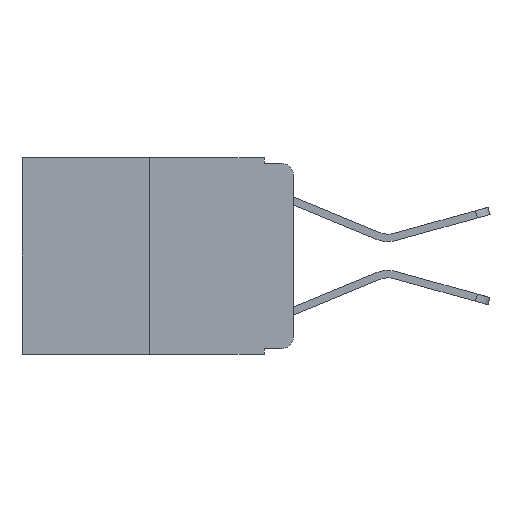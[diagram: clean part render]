
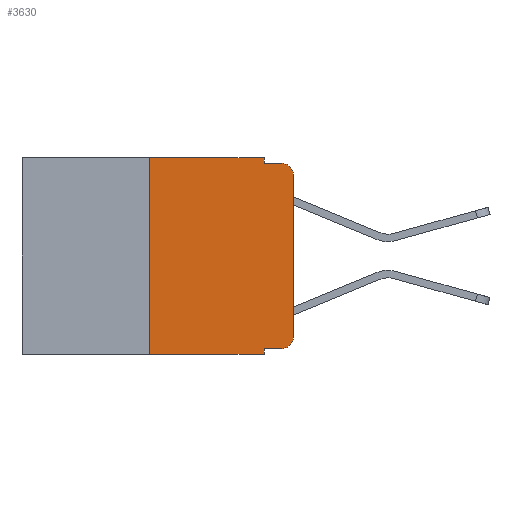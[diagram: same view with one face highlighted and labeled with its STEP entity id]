
A CAD part, left-side view. The second image highlights one B-rep face of the part: STEP entity #3630.
In plain terms, the highlighted planar face has unit normal (-1, 0, 0).
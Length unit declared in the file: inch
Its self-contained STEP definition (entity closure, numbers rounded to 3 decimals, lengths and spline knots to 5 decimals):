
#124 = CIRCLE ( 'NONE', #5403, 0.02 ) ;
#1052 = CARTESIAN_POINT ( 'NONE',  ( 0., 0.051, -0.333 ) ) ;
#1089 = DIRECTION ( 'NONE',  ( 0., -1., 0. ) ) ;
#1124 = ORIENTED_EDGE ( 'NONE', *, *, #21594, .F. ) ;
#1941 = VECTOR ( 'NONE', #14794, 39.37008 ) ;
#1999 = ORIENTED_EDGE ( 'NONE', *, *, #22558, .T. ) ;
#2026 = ORIENTED_EDGE ( 'NONE', *, *, #15495, .T. ) ;
#2114 = VERTEX_POINT ( 'NONE', #12562 ) ;
#2465 = FACE_OUTER_BOUND ( 'NONE', #10797, .T. ) ;
#2575 = AXIS2_PLACEMENT_3D ( 'NONE', #5648, #18762, #7581 ) ;
#2713 = ORIENTED_EDGE ( 'NONE', *, *, #6636, .F. ) ;
#2797 = VECTOR ( 'NONE', #1089, 39.37008 ) ;
#2868 = VERTEX_POINT ( 'NONE', #6499 ) ;
#3630 = ADVANCED_FACE ( 'NONE', ( #2465 ), #11433, .F. ) ;
#4038 = ORIENTED_EDGE ( 'NONE', *, *, #5647, .F. ) ;
#4309 = CARTESIAN_POINT ( 'NONE',  ( 0., 0.051, 0. ) ) ;
#4724 = CARTESIAN_POINT ( 'NONE',  ( 0., 0.25, 0. ) ) ;
#4767 = CARTESIAN_POINT ( 'NONE',  ( 0., 0., -0.03 ) ) ;
#5021 = DIRECTION ( 'NONE',  ( 0., -1., 0. ) ) ;
#5087 = ORIENTED_EDGE ( 'NONE', *, *, #15776, .T. ) ;
#5118 = LINE ( 'NONE', #15468, #9636 ) ;
#5278 = VERTEX_POINT ( 'NONE', #1052 ) ;
#5403 = AXIS2_PLACEMENT_3D ( 'NONE', #8069, #21046, #9980 ) ;
#5580 = VERTEX_POINT ( 'NONE', #20873 ) ;
#5647 = EDGE_CURVE ( 'NONE', #14646, #10411, #5118, .T. ) ;
#5648 = CARTESIAN_POINT ( 'NONE',  ( 0., 0.02, -0.03 ) ) ;
#5752 = ORIENTED_EDGE ( 'NONE', *, *, #6747, .F. ) ;
#6122 = DIRECTION ( 'NONE',  ( 0., 0., -1. ) ) ;
#6426 = CARTESIAN_POINT ( 'NONE',  ( 0., 0.473, -0.343 ) ) ;
#6499 = CARTESIAN_POINT ( 'NONE',  ( 0., 0., -0.313 ) ) ;
#6636 = EDGE_CURVE ( 'NONE', #5580, #12687, #10323, .T. ) ;
#6747 = EDGE_CURVE ( 'NONE', #10411, #2114, #13504, .T. ) ;
#6860 = AXIS2_PLACEMENT_3D ( 'NONE', #7709, #11502, #24369 ) ;
#7247 = LINE ( 'NONE', #21085, #11660 ) ;
#7581 = DIRECTION ( 'NONE',  ( 0., 0., -1. ) ) ;
#7709 = CARTESIAN_POINT ( 'NONE',  ( 0., 0.473, 0. ) ) ;
#7804 = VECTOR ( 'NONE', #20015, 39.37008 ) ;
#8069 = CARTESIAN_POINT ( 'NONE',  ( 0., 0.02, -0.313 ) ) ;
#8228 = CARTESIAN_POINT ( 'NONE',  ( 0., 0.051, -0.01 ) ) ;
#8314 = CARTESIAN_POINT ( 'NONE',  ( 0., 0.02, -0.333 ) ) ;
#9636 = VECTOR ( 'NONE', #6122, 39.37008 ) ;
#9980 = DIRECTION ( 'NONE',  ( 0., 0., -1. ) ) ;
#10142 = VECTOR ( 'NONE', #5021, 39.37008 ) ;
#10323 = LINE ( 'NONE', #4724, #14672 ) ;
#10411 = VERTEX_POINT ( 'NONE', #8228 ) ;
#10477 = VERTEX_POINT ( 'NONE', #8314 ) ;
#10779 = CARTESIAN_POINT ( 'NONE',  ( 0., 0.051, -0.333 ) ) ;
#10797 = EDGE_LOOP ( 'NONE', ( #12908, #17136, #5752, #4038, #1124, #2713, #1999, #21776, #5087, #2026 ) ) ;
#11068 = CARTESIAN_POINT ( 'NONE',  ( 0., 0., 0. ) ) ;
#11326 = CARTESIAN_POINT ( 'NONE',  ( 0., 0.25, 0. ) ) ;
#11433 = PLANE ( 'NONE',  #6860 ) ;
#11502 = DIRECTION ( 'NONE',  ( 1., 0., 0. ) ) ;
#11660 = VECTOR ( 'NONE', #11879, 39.37008 ) ;
#11879 = DIRECTION ( 'NONE',  ( 0., 0., -1. ) ) ;
#12562 = CARTESIAN_POINT ( 'NONE',  ( 0., 0.02, -0.01 ) ) ;
#12687 = VERTEX_POINT ( 'NONE', #11326 ) ;
#12755 = LINE ( 'NONE', #11068, #1941 ) ;
#12814 = LINE ( 'NONE', #10779, #7804 ) ;
#12908 = ORIENTED_EDGE ( 'NONE', *, *, #17805, .T. ) ;
#13344 = VERTEX_POINT ( 'NONE', #19337 ) ;
#13504 = LINE ( 'NONE', #14462, #2797 ) ;
#14141 = VERTEX_POINT ( 'NONE', #4767 ) ;
#14462 = CARTESIAN_POINT ( 'NONE',  ( 0., 0.051, -0.01 ) ) ;
#14646 = VERTEX_POINT ( 'NONE', #4309 ) ;
#14672 = VECTOR ( 'NONE', #15994, 39.37008 ) ;
#14794 = DIRECTION ( 'NONE',  ( 0., 0., 1. ) ) ;
#15468 = CARTESIAN_POINT ( 'NONE',  ( 0., 0.051, 0. ) ) ;
#15495 = EDGE_CURVE ( 'NONE', #10477, #2868, #124, .T. ) ;
#15776 = EDGE_CURVE ( 'NONE', #5278, #10477, #12814, .T. ) ;
#15994 = DIRECTION ( 'NONE',  ( 0., 0., 1. ) ) ;
#17136 = ORIENTED_EDGE ( 'NONE', *, *, #22873, .T. ) ;
#17805 = EDGE_CURVE ( 'NONE', #2868, #14141, #12755, .T. ) ;
#18239 = CARTESIAN_POINT ( 'NONE',  ( 0., 0.473, 0. ) ) ;
#18762 = DIRECTION ( 'NONE',  ( -1., 0., 0. ) ) ;
#19337 = CARTESIAN_POINT ( 'NONE',  ( 0., 0.051, -0.343 ) ) ;
#19350 = EDGE_CURVE ( 'NONE', #5278, #13344, #7247, .T. ) ;
#19588 = DIRECTION ( 'NONE',  ( 0., -1., 0. ) ) ;
#20002 = LINE ( 'NONE', #18239, #10142 ) ;
#20015 = DIRECTION ( 'NONE',  ( 0., -1., 0. ) ) ;
#20873 = CARTESIAN_POINT ( 'NONE',  ( 0., 0.25, -0.343 ) ) ;
#21046 = DIRECTION ( 'NONE',  ( -1., 0., 0. ) ) ;
#21085 = CARTESIAN_POINT ( 'NONE',  ( 0., 0.051, 0. ) ) ;
#21349 = VECTOR ( 'NONE', #19588, 39.37008 ) ;
#21594 = EDGE_CURVE ( 'NONE', #12687, #14646, #20002, .T. ) ;
#21776 = ORIENTED_EDGE ( 'NONE', *, *, #19350, .F. ) ;
#21933 = LINE ( 'NONE', #6426, #21349 ) ;
#22558 = EDGE_CURVE ( 'NONE', #5580, #13344, #21933, .T. ) ;
#22873 = EDGE_CURVE ( 'NONE', #14141, #2114, #24179, .T. ) ;
#24179 = CIRCLE ( 'NONE', #2575, 0.02 ) ;
#24369 = DIRECTION ( 'NONE',  ( 0., 0., -1. ) ) ;
